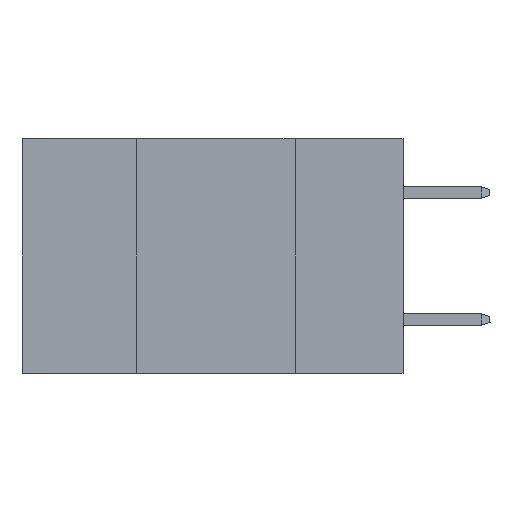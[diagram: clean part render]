
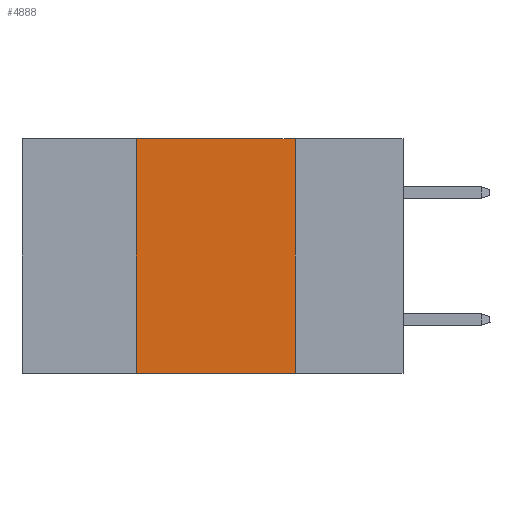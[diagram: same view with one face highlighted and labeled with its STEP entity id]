
A CAD part, left-side view. The second image highlights one B-rep face of the part: STEP entity #4888.
In plain terms, the highlighted planar face has unit normal (-1, 0, 0).
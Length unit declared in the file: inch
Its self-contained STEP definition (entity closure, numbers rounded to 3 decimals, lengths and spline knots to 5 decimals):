
#2397 = LINE ( 'NONE', #2558, #31285 ) ;
#2550 = LINE ( 'NONE', #20613, #13278 ) ;
#2558 = CARTESIAN_POINT ( 'NONE',  ( 0., 0.17, 0. ) ) ;
#4888 = ADVANCED_FACE ( 'NONE', ( #11099 ), #8502, .F. ) ;
#5750 = DIRECTION ( 'NONE',  ( 0., 0., -1. ) ) ;
#6311 = VERTEX_POINT ( 'NONE', #9701 ) ;
#6375 = CARTESIAN_POINT ( 'NONE',  ( 0., 0.6, 0. ) ) ;
#6451 = AXIS2_PLACEMENT_3D ( 'NONE', #6375, #28441, #5750 ) ;
#6786 = ORIENTED_EDGE ( 'NONE', *, *, #13386, .F. ) ;
#7120 = LINE ( 'NONE', #11708, #7590 ) ;
#7590 = VECTOR ( 'NONE', #9408, 39.37008 ) ;
#8502 = PLANE ( 'NONE',  #6451 ) ;
#9408 = DIRECTION ( 'NONE',  ( 0., -1., 0. ) ) ;
#9701 = CARTESIAN_POINT ( 'NONE',  ( 0., 0.42, -0.37 ) ) ;
#10846 = CARTESIAN_POINT ( 'NONE',  ( 0., 0.17, -0.37 ) ) ;
#11099 = FACE_OUTER_BOUND ( 'NONE', #20846, .T. ) ;
#11236 = ORIENTED_EDGE ( 'NONE', *, *, #31363, .F. ) ;
#11708 = CARTESIAN_POINT ( 'NONE',  ( 0., 0.6, 0. ) ) ;
#11984 = CARTESIAN_POINT ( 'NONE',  ( 0., 0.42, 0. ) ) ;
#12209 = EDGE_CURVE ( 'NONE', #6311, #25614, #22031, .T. ) ;
#12323 = DIRECTION ( 'NONE',  ( 0., 0., 1. ) ) ;
#12888 = DIRECTION ( 'NONE',  ( 0., -1., 0. ) ) ;
#13278 = VECTOR ( 'NONE', #12888, 39.37008 ) ;
#13386 = EDGE_CURVE ( 'NONE', #25614, #14515, #7120, .T. ) ;
#14501 = EDGE_CURVE ( 'NONE', #6311, #22986, #2550, .T. ) ;
#14515 = VERTEX_POINT ( 'NONE', #22916 ) ;
#16790 = ORIENTED_EDGE ( 'NONE', *, *, #14501, .T. ) ;
#17526 = ORIENTED_EDGE ( 'NONE', *, *, #12209, .F. ) ;
#20613 = CARTESIAN_POINT ( 'NONE',  ( 0., 0.6, -0.37 ) ) ;
#20840 = VECTOR ( 'NONE', #12323, 39.37008 ) ;
#20846 = EDGE_LOOP ( 'NONE', ( #11236, #6786, #17526, #16790 ) ) ;
#22031 = LINE ( 'NONE', #11984, #20840 ) ;
#22302 = DIRECTION ( 'NONE',  ( 0., 0., -1. ) ) ;
#22819 = CARTESIAN_POINT ( 'NONE',  ( 0., 0.42, 0. ) ) ;
#22916 = CARTESIAN_POINT ( 'NONE',  ( 0., 0.17, 0. ) ) ;
#22986 = VERTEX_POINT ( 'NONE', #10846 ) ;
#25614 = VERTEX_POINT ( 'NONE', #22819 ) ;
#28441 = DIRECTION ( 'NONE',  ( 1., 0., 0. ) ) ;
#31285 = VECTOR ( 'NONE', #22302, 39.37008 ) ;
#31363 = EDGE_CURVE ( 'NONE', #14515, #22986, #2397, .T. ) ;
